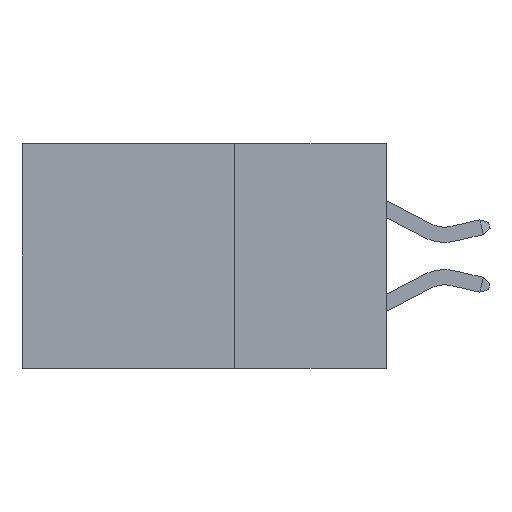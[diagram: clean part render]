
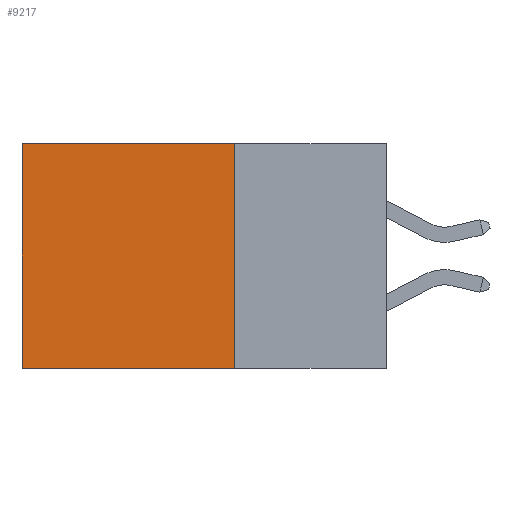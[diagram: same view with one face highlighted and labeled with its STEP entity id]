
A CAD part, left-side view. The second image highlights one B-rep face of the part: STEP entity #9217.
In plain terms, the highlighted planar face has unit normal (-1, 0, 0).
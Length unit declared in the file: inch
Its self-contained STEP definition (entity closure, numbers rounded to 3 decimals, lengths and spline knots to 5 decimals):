
#364 = CARTESIAN_POINT ( 'NONE',  ( 0.298, 0.6, 0. ) ) ;
#479 = LINE ( 'NONE', #7746, #3609 ) ;
#1082 = DIRECTION ( 'NONE',  ( 0., 0., -1. ) ) ;
#1167 = VECTOR ( 'NONE', #1082, 39.37008 ) ;
#1239 = VERTEX_POINT ( 'NONE', #1771 ) ;
#1435 = LINE ( 'NONE', #9321, #8388 ) ;
#1771 = CARTESIAN_POINT ( 'NONE',  ( 0.298, 0.25, 0. ) ) ;
#1873 = VERTEX_POINT ( 'NONE', #12087 ) ;
#2414 = ORIENTED_EDGE ( 'NONE', *, *, #4961, .F. ) ;
#2425 = AXIS2_PLACEMENT_3D ( 'NONE', #10470, #4881, #11386 ) ;
#2842 = VECTOR ( 'NONE', #4608, 39.37008 ) ;
#3160 = VERTEX_POINT ( 'NONE', #9354 ) ;
#3312 = ORIENTED_EDGE ( 'NONE', *, *, #7510, .F. ) ;
#3609 = VECTOR ( 'NONE', #8662, 39.37008 ) ;
#3645 = CARTESIAN_POINT ( 'NONE',  ( 0.298, 0.6, 0. ) ) ;
#3712 = LINE ( 'NONE', #9528, #1167 ) ;
#3921 = PLANE ( 'NONE',  #2425 ) ;
#4608 = DIRECTION ( 'NONE',  ( 0., 0., -1. ) ) ;
#4660 = DIRECTION ( 'NONE',  ( 0., 1., 0. ) ) ;
#4881 = DIRECTION ( 'NONE',  ( 1., 0., 0. ) ) ;
#4961 = EDGE_CURVE ( 'NONE', #3160, #1873, #479, .T. ) ;
#5522 = EDGE_LOOP ( 'NONE', ( #10698, #2414, #3312, #11617 ) ) ;
#6308 = EDGE_CURVE ( 'NONE', #11211, #1873, #10354, .T. ) ;
#7417 = FACE_OUTER_BOUND ( 'NONE', #5522, .T. ) ;
#7510 = EDGE_CURVE ( 'NONE', #1239, #3160, #3712, .T. ) ;
#7746 = CARTESIAN_POINT ( 'NONE',  ( 0.298, 0.25, -0.37 ) ) ;
#8388 = VECTOR ( 'NONE', #4660, 39.37008 ) ;
#8662 = DIRECTION ( 'NONE',  ( 0., 1., 0. ) ) ;
#9217 = ADVANCED_FACE ( 'NONE', ( #7417 ), #3921, .F. ) ;
#9321 = CARTESIAN_POINT ( 'NONE',  ( 0.298, 0.25, 0. ) ) ;
#9354 = CARTESIAN_POINT ( 'NONE',  ( 0.298, 0.25, -0.37 ) ) ;
#9528 = CARTESIAN_POINT ( 'NONE',  ( 0.298, 0.25, 0. ) ) ;
#9771 = EDGE_CURVE ( 'NONE', #1239, #11211, #1435, .T. ) ;
#10354 = LINE ( 'NONE', #3645, #2842 ) ;
#10470 = CARTESIAN_POINT ( 'NONE',  ( 0.298, 0.25, 0. ) ) ;
#10698 = ORIENTED_EDGE ( 'NONE', *, *, #6308, .T. ) ;
#11211 = VERTEX_POINT ( 'NONE', #364 ) ;
#11386 = DIRECTION ( 'NONE',  ( 0., 0., -1. ) ) ;
#11617 = ORIENTED_EDGE ( 'NONE', *, *, #9771, .T. ) ;
#12087 = CARTESIAN_POINT ( 'NONE',  ( 0.298, 0.6, -0.37 ) ) ;
